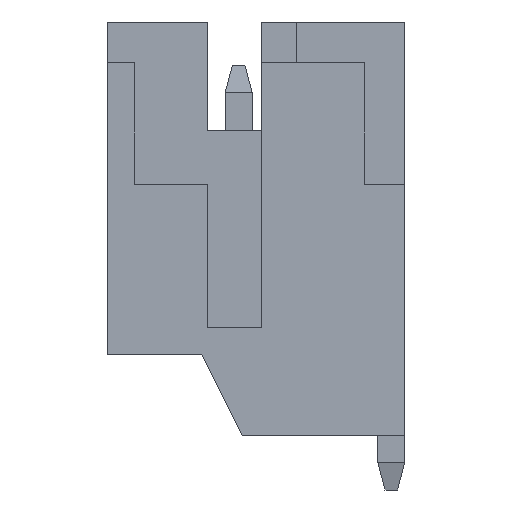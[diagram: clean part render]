
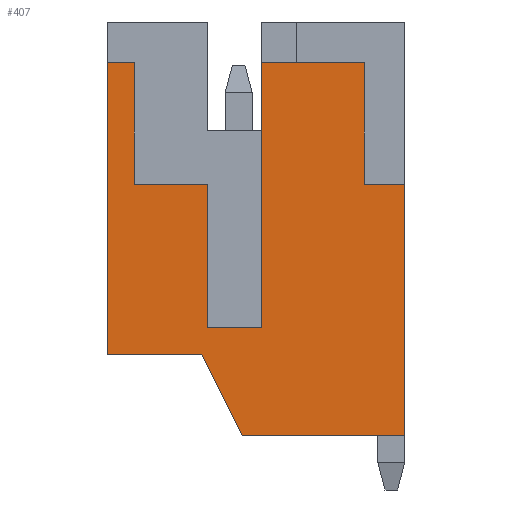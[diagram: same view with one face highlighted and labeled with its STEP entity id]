
A CAD part, left-side view. The second image highlights one B-rep face of the part: STEP entity #407.
In plain terms, the highlighted planar face has unit normal (-1, 0, 0).
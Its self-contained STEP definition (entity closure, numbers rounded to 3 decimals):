
#37 = VECTOR ( 'NONE', #6369, 1000. ) ;
#40 = VECTOR ( 'NONE', #6441, 1000. ) ;
#171 = ORIENTED_EDGE ( 'NONE', *, *, #1731, .T. ) ;
#337 = CARTESIAN_POINT ( 'NONE',  ( -3., -0.07, -1.5 ) ) ;
#347 = ORIENTED_EDGE ( 'NONE', *, *, #1249, .F. ) ;
#407 = ADVANCED_FACE ( 'NONE', ( #4328 ), #7078, .T. ) ;
#455 = VECTOR ( 'NONE', #5655, 1000. ) ;
#649 = VERTEX_POINT ( 'NONE', #7224 ) ;
#767 = VERTEX_POINT ( 'NONE', #4262 ) ;
#954 = DIRECTION ( 'NONE',  ( 0., -1., 0. ) ) ;
#999 = ORIENTED_EDGE ( 'NONE', *, *, #6992, .T. ) ;
#1192 = CARTESIAN_POINT ( 'NONE',  ( -3., -2.32, 5.4 ) ) ;
#1244 = CARTESIAN_POINT ( 'NONE',  ( -3., 0.58, 0.5 ) ) ;
#1249 = EDGE_CURVE ( 'NONE', #4447, #3377, #4505, .T. ) ;
#1292 = LINE ( 'NONE', #5610, #6898 ) ;
#1350 = VECTOR ( 'NONE', #4279, 1000. ) ;
#1366 = LINE ( 'NONE', #2703, #4618 ) ;
#1395 = ORIENTED_EDGE ( 'NONE', *, *, #2430, .T. ) ;
#1450 = CARTESIAN_POINT ( 'NONE',  ( -3., 1.93, 3.15 ) ) ;
#1596 = AXIS2_PLACEMENT_3D ( 'NONE', #1947, #1973, #2118 ) ;
#1717 = VERTEX_POINT ( 'NONE', #1450 ) ;
#1731 = EDGE_CURVE ( 'NONE', #3666, #7894, #5449, .T. ) ;
#1742 = CARTESIAN_POINT ( 'NONE',  ( -3., -2.32, 3.15 ) ) ;
#1830 = CARTESIAN_POINT ( 'NONE',  ( -3., 1.93, 3.15 ) ) ;
#1878 = VERTEX_POINT ( 'NONE', #4968 ) ;
#1947 = CARTESIAN_POINT ( 'NONE',  ( -3., 0., 0. ) ) ;
#1973 = DIRECTION ( 'NONE',  ( -1., 0., 0. ) ) ;
#2079 = CARTESIAN_POINT ( 'NONE',  ( -3., -0.42, 5.4 ) ) ;
#2103 = VECTOR ( 'NONE', #7979, 1000. ) ;
#2118 = DIRECTION ( 'NONE',  ( 0., -1., 0. ) ) ;
#2162 = CARTESIAN_POINT ( 'NONE',  ( -3., -0.42, 0.5 ) ) ;
#2272 = VERTEX_POINT ( 'NONE', #1742 ) ;
#2290 = ORIENTED_EDGE ( 'NONE', *, *, #6259, .F. ) ;
#2398 = DIRECTION ( 'NONE',  ( 0., -1., 0. ) ) ;
#2430 = EDGE_CURVE ( 'NONE', #7880, #649, #1292, .T. ) ;
#2509 = VERTEX_POINT ( 'NONE', #5708 ) ;
#2703 = CARTESIAN_POINT ( 'NONE',  ( -3., -3.07, 5.4 ) ) ;
#2764 = EDGE_LOOP ( 'NONE', ( #171, #6139, #2849, #999, #1395, #2851, #3088, #7794, #7500, #3153, #347, #5102, #2290, #5680 ) ) ;
#2829 = EDGE_CURVE ( 'NONE', #767, #2509, #7867, .T. ) ;
#2849 = ORIENTED_EDGE ( 'NONE', *, *, #2829, .T. ) ;
#2851 = ORIENTED_EDGE ( 'NONE', *, *, #7040, .T. ) ;
#2943 = CARTESIAN_POINT ( 'NONE',  ( -3., 1.93, 5.4 ) ) ;
#2966 = VECTOR ( 'NONE', #8088, 1000. ) ;
#3070 = DIRECTION ( 'NONE',  ( 0., 0., -1. ) ) ;
#3080 = CARTESIAN_POINT ( 'NONE',  ( -3., -3.07, 6.15 ) ) ;
#3088 = ORIENTED_EDGE ( 'NONE', *, *, #7830, .F. ) ;
#3153 = ORIENTED_EDGE ( 'NONE', *, *, #7396, .T. ) ;
#3161 = CARTESIAN_POINT ( 'NONE',  ( -3., -3.07, 3.15 ) ) ;
#3227 = DIRECTION ( 'NONE',  ( 0., 1., 0. ) ) ;
#3312 = EDGE_CURVE ( 'NONE', #1878, #4447, #7268, .T. ) ;
#3377 = VERTEX_POINT ( 'NONE', #7567 ) ;
#3602 = CARTESIAN_POINT ( 'NONE',  ( -3., -0.42, 6.15 ) ) ;
#3617 = EDGE_CURVE ( 'NONE', #6240, #5795, #1366, .T. ) ;
#3666 = VERTEX_POINT ( 'NONE', #2943 ) ;
#3782 = LINE ( 'NONE', #6828, #455 ) ;
#3831 = VECTOR ( 'NONE', #3070, 1000. ) ;
#3845 = VERTEX_POINT ( 'NONE', #3161 ) ;
#4262 = CARTESIAN_POINT ( 'NONE',  ( -3., 2.43, 0. ) ) ;
#4279 = DIRECTION ( 'NONE',  ( 0., 0., 1. ) ) ;
#4328 = FACE_OUTER_BOUND ( 'NONE', #2764, .T. ) ;
#4361 = LINE ( 'NONE', #7634, #37 ) ;
#4447 = VERTEX_POINT ( 'NONE', #1244 ) ;
#4491 = DIRECTION ( 'NONE',  ( 0., -1., 0. ) ) ;
#4505 = LINE ( 'NONE', #2162, #7438 ) ;
#4584 = EDGE_CURVE ( 'NONE', #7894, #767, #6554, .T. ) ;
#4596 = LINE ( 'NONE', #6759, #1350 ) ;
#4618 = VECTOR ( 'NONE', #3227, 1000. ) ;
#4744 = VECTOR ( 'NONE', #4940, 1000. ) ;
#4897 = EDGE_CURVE ( 'NONE', #2272, #6240, #4596, .T. ) ;
#4940 = DIRECTION ( 'NONE',  ( 0., 0., 1. ) ) ;
#4948 = CARTESIAN_POINT ( 'NONE',  ( -3., 0.58, 3.15 ) ) ;
#4952 = LINE ( 'NONE', #3080, #2966 ) ;
#4954 = VECTOR ( 'NONE', #5952, 1000. ) ;
#4968 = CARTESIAN_POINT ( 'NONE',  ( -3., 0.58, 3.15 ) ) ;
#5102 = ORIENTED_EDGE ( 'NONE', *, *, #3312, .F. ) ;
#5180 = CARTESIAN_POINT ( 'NONE',  ( -3., 2.43, 0. ) ) ;
#5185 = CARTESIAN_POINT ( 'NONE',  ( -3., 2.43, 6.15 ) ) ;
#5285 = CARTESIAN_POINT ( 'NONE',  ( -3., -2.32, 3.15 ) ) ;
#5449 = LINE ( 'NONE', #7096, #40 ) ;
#5490 = VECTOR ( 'NONE', #7691, 1000. ) ;
#5610 = CARTESIAN_POINT ( 'NONE',  ( -3., -3.07, -1.5 ) ) ;
#5655 = DIRECTION ( 'NONE',  ( 0., -1., 0. ) ) ;
#5680 = ORIENTED_EDGE ( 'NONE', *, *, #8085, .T. ) ;
#5708 = CARTESIAN_POINT ( 'NONE',  ( -3., 0.68, 0. ) ) ;
#5795 = VERTEX_POINT ( 'NONE', #2079 ) ;
#5802 = VECTOR ( 'NONE', #4491, 1000. ) ;
#5952 = DIRECTION ( 'NONE',  ( 0., -1., 0. ) ) ;
#6139 = ORIENTED_EDGE ( 'NONE', *, *, #4584, .T. ) ;
#6240 = VERTEX_POINT ( 'NONE', #1192 ) ;
#6259 = EDGE_CURVE ( 'NONE', #1717, #1878, #3782, .T. ) ;
#6369 = DIRECTION ( 'NONE',  ( 0., -0.447, -0.894 ) ) ;
#6441 = DIRECTION ( 'NONE',  ( 0., 1., 0. ) ) ;
#6554 = LINE ( 'NONE', #5185, #5490 ) ;
#6600 = LINE ( 'NONE', #1830, #4744 ) ;
#6605 = CARTESIAN_POINT ( 'NONE',  ( -3., 2.43, 5.4 ) ) ;
#6759 = CARTESIAN_POINT ( 'NONE',  ( -3., -2.32, 3.15 ) ) ;
#6828 = CARTESIAN_POINT ( 'NONE',  ( -3., -0.42, 3.15 ) ) ;
#6898 = VECTOR ( 'NONE', #2398, 1000. ) ;
#6992 = EDGE_CURVE ( 'NONE', #2509, #7880, #4361, .T. ) ;
#7040 = EDGE_CURVE ( 'NONE', #649, #3845, #4952, .T. ) ;
#7078 = PLANE ( 'NONE',  #1596 ) ;
#7096 = CARTESIAN_POINT ( 'NONE',  ( -3., -3.07, 5.4 ) ) ;
#7105 = LINE ( 'NONE', #5285, #4954 ) ;
#7224 = CARTESIAN_POINT ( 'NONE',  ( -3., -3.07, -1.5 ) ) ;
#7268 = LINE ( 'NONE', #4948, #3831 ) ;
#7396 = EDGE_CURVE ( 'NONE', #5795, #3377, #7496, .T. ) ;
#7438 = VECTOR ( 'NONE', #954, 1000. ) ;
#7496 = LINE ( 'NONE', #3602, #2103 ) ;
#7500 = ORIENTED_EDGE ( 'NONE', *, *, #3617, .T. ) ;
#7567 = CARTESIAN_POINT ( 'NONE',  ( -3., -0.42, 0.5 ) ) ;
#7634 = CARTESIAN_POINT ( 'NONE',  ( -3., -0.07, -1.5 ) ) ;
#7691 = DIRECTION ( 'NONE',  ( 0., 0., -1. ) ) ;
#7794 = ORIENTED_EDGE ( 'NONE', *, *, #4897, .T. ) ;
#7830 = EDGE_CURVE ( 'NONE', #2272, #3845, #7105, .T. ) ;
#7867 = LINE ( 'NONE', #5180, #5802 ) ;
#7880 = VERTEX_POINT ( 'NONE', #337 ) ;
#7894 = VERTEX_POINT ( 'NONE', #6605 ) ;
#7979 = DIRECTION ( 'NONE',  ( 0., 0., -1. ) ) ;
#8085 = EDGE_CURVE ( 'NONE', #1717, #3666, #6600, .T. ) ;
#8088 = DIRECTION ( 'NONE',  ( 0., 0., 1. ) ) ;
